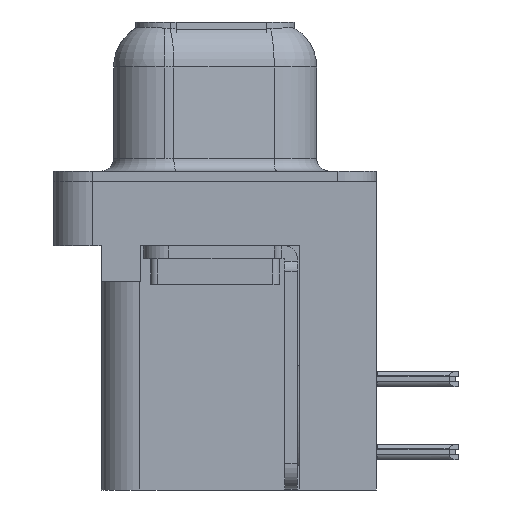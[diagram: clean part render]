
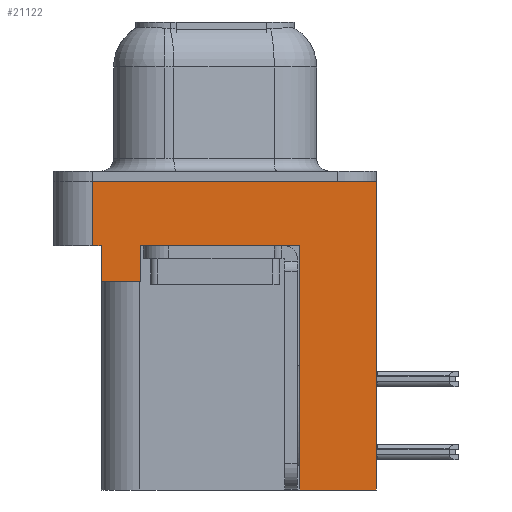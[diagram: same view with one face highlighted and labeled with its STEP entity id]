
A CAD part, left-side view. The second image highlights one B-rep face of the part: STEP entity #21122.
In plain terms, the highlighted planar face has unit normal (-1, 0, 0).
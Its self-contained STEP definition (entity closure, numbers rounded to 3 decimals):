
#1592 = LINE ( 'NONE', #31117, #31879 ) ;
#1787 = LINE ( 'NONE', #28203, #20670 ) ;
#2267 = ORIENTED_EDGE ( 'NONE', *, *, #22909, .F. ) ;
#2482 = DIRECTION ( 'NONE',  ( 0., -1., 0. ) ) ;
#2527 = CARTESIAN_POINT ( 'NONE',  ( -3., 4.775, 0. ) ) ;
#3108 = LINE ( 'NONE', #7544, #13303 ) ;
#3486 = CARTESIAN_POINT ( 'NONE',  ( -3., 4.775, -2.5 ) ) ;
#3587 = VERTEX_POINT ( 'NONE', #9784 ) ;
#4604 = LINE ( 'NONE', #11589, #21929 ) ;
#5018 = ORIENTED_EDGE ( 'NONE', *, *, #29088, .T. ) ;
#5254 = ORIENTED_EDGE ( 'NONE', *, *, #27159, .F. ) ;
#5550 = VERTEX_POINT ( 'NONE', #19767 ) ;
#5709 = EDGE_CURVE ( 'NONE', #21786, #10015, #31665, .T. ) ;
#6416 = ORIENTED_EDGE ( 'NONE', *, *, #7354, .T. ) ;
#6657 = CARTESIAN_POINT ( 'NONE',  ( -3., -3.295, -12. ) ) ;
#6772 = CARTESIAN_POINT ( 'NONE',  ( -3., 2.895, -3.9 ) ) ;
#6825 = LINE ( 'NONE', #7634, #13883 ) ;
#7123 = DIRECTION ( 'NONE',  ( 0., 0., 1. ) ) ;
#7231 = ORIENTED_EDGE ( 'NONE', *, *, #26785, .F. ) ;
#7282 = VERTEX_POINT ( 'NONE', #12024 ) ;
#7354 = EDGE_CURVE ( 'NONE', #10015, #16778, #22160, .T. ) ;
#7544 = CARTESIAN_POINT ( 'NONE',  ( -3., -3.295, -12. ) ) ;
#7634 = CARTESIAN_POINT ( 'NONE',  ( -3., -6.275, -2.5 ) ) ;
#8756 = VECTOR ( 'NONE', #16344, 1000. ) ;
#8856 = EDGE_LOOP ( 'NONE', ( #30241, #32439, #5018, #22520, #2267, #16172, #6416, #7231, #5254, #20959 ) ) ;
#9505 = CARTESIAN_POINT ( 'NONE',  ( -3., 4.425, -2.5 ) ) ;
#9634 = VECTOR ( 'NONE', #17524, 1000. ) ;
#9784 = CARTESIAN_POINT ( 'NONE',  ( -3., -3.295, -12. ) ) ;
#10015 = VERTEX_POINT ( 'NONE', #14272 ) ;
#10507 = LINE ( 'NONE', #6657, #18002 ) ;
#10711 = DIRECTION ( 'NONE',  ( 0., 0., 1. ) ) ;
#11509 = LINE ( 'NONE', #21346, #8756 ) ;
#11589 = CARTESIAN_POINT ( 'NONE',  ( -3., -6.275, 0. ) ) ;
#11902 = CARTESIAN_POINT ( 'NONE',  ( -3., -3.295, -2.5 ) ) ;
#12024 = CARTESIAN_POINT ( 'NONE',  ( -3., -6.275, 0. ) ) ;
#12978 = FACE_OUTER_BOUND ( 'NONE', #8856, .T. ) ;
#13303 = VECTOR ( 'NONE', #7123, 1000. ) ;
#13584 = AXIS2_PLACEMENT_3D ( 'NONE', #19007, #18543, #24289 ) ;
#13883 = VECTOR ( 'NONE', #15355, 1000. ) ;
#14272 = CARTESIAN_POINT ( 'NONE',  ( -3., 2.895, -2.5 ) ) ;
#15253 = CARTESIAN_POINT ( 'NONE',  ( -3., 4.775, -2.5 ) ) ;
#15355 = DIRECTION ( 'NONE',  ( 0., 0., 1. ) ) ;
#15674 = CARTESIAN_POINT ( 'NONE',  ( -3., 4.425, -3.9 ) ) ;
#16172 = ORIENTED_EDGE ( 'NONE', *, *, #5709, .T. ) ;
#16344 = DIRECTION ( 'NONE',  ( 0., -1., 0. ) ) ;
#16778 = VERTEX_POINT ( 'NONE', #11902 ) ;
#17524 = DIRECTION ( 'NONE',  ( 0., 0., 1. ) ) ;
#18002 = VECTOR ( 'NONE', #21313, 1000. ) ;
#18543 = DIRECTION ( 'NONE',  ( -1., 0., 0. ) ) ;
#18644 = DIRECTION ( 'NONE',  ( 0., 0., 1. ) ) ;
#18792 = EDGE_CURVE ( 'NONE', #28183, #31058, #1787, .T. ) ;
#19007 = CARTESIAN_POINT ( 'NONE',  ( -3., -6.275, -2.5 ) ) ;
#19244 = EDGE_CURVE ( 'NONE', #5550, #7282, #6825, .T. ) ;
#19767 = CARTESIAN_POINT ( 'NONE',  ( -3., -6.275, -12. ) ) ;
#20470 = VECTOR ( 'NONE', #18644, 1000. ) ;
#20670 = VECTOR ( 'NONE', #10711, 1000. ) ;
#20959 = ORIENTED_EDGE ( 'NONE', *, *, #19244, .T. ) ;
#21122 = ADVANCED_FACE ( 'NONE', ( #12978 ), #26376, .T. ) ;
#21313 = DIRECTION ( 'NONE',  ( 0., 1., 0. ) ) ;
#21346 = CARTESIAN_POINT ( 'NONE',  ( -3., -6.275, -2.5 ) ) ;
#21786 = VERTEX_POINT ( 'NONE', #6772 ) ;
#21929 = VECTOR ( 'NONE', #26580, 1000. ) ;
#22160 = LINE ( 'NONE', #25221, #23714 ) ;
#22520 = ORIENTED_EDGE ( 'NONE', *, *, #18792, .F. ) ;
#22909 = EDGE_CURVE ( 'NONE', #21786, #28183, #1592, .T. ) ;
#23714 = VECTOR ( 'NONE', #2482, 1000. ) ;
#24289 = DIRECTION ( 'NONE',  ( 0., 0., 1. ) ) ;
#25221 = CARTESIAN_POINT ( 'NONE',  ( -3., -6.275, -2.5 ) ) ;
#26376 = PLANE ( 'NONE',  #13584 ) ;
#26423 = DIRECTION ( 'NONE',  ( 0., 1., 0. ) ) ;
#26580 = DIRECTION ( 'NONE',  ( 0., -1., 0. ) ) ;
#26741 = VERTEX_POINT ( 'NONE', #2527 ) ;
#26785 = EDGE_CURVE ( 'NONE', #3587, #16778, #3108, .T. ) ;
#27159 = EDGE_CURVE ( 'NONE', #5550, #3587, #10507, .T. ) ;
#28183 = VERTEX_POINT ( 'NONE', #15674 ) ;
#28203 = CARTESIAN_POINT ( 'NONE',  ( -3., 4.425, -3.9 ) ) ;
#28253 = EDGE_CURVE ( 'NONE', #26741, #7282, #4604, .T. ) ;
#29088 = EDGE_CURVE ( 'NONE', #31998, #31058, #11509, .T. ) ;
#30087 = EDGE_CURVE ( 'NONE', #31998, #26741, #30291, .T. ) ;
#30241 = ORIENTED_EDGE ( 'NONE', *, *, #28253, .F. ) ;
#30291 = LINE ( 'NONE', #3486, #20470 ) ;
#31058 = VERTEX_POINT ( 'NONE', #9505 ) ;
#31117 = CARTESIAN_POINT ( 'NONE',  ( -3., 4.425, -3.9 ) ) ;
#31665 = LINE ( 'NONE', #32093, #9634 ) ;
#31879 = VECTOR ( 'NONE', #26423, 1000. ) ;
#31998 = VERTEX_POINT ( 'NONE', #15253 ) ;
#32093 = CARTESIAN_POINT ( 'NONE',  ( -3., 2.895, -3.9 ) ) ;
#32439 = ORIENTED_EDGE ( 'NONE', *, *, #30087, .F. ) ;
